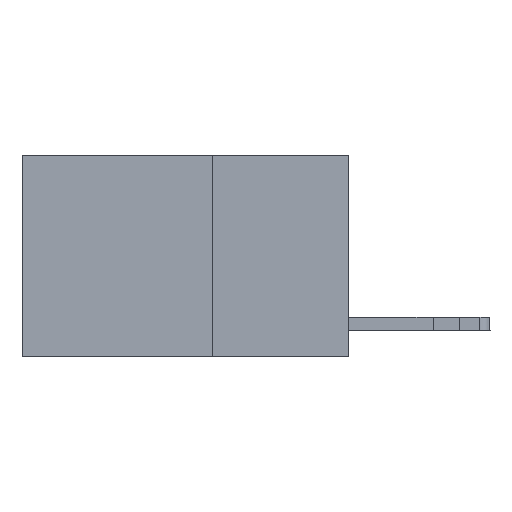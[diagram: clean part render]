
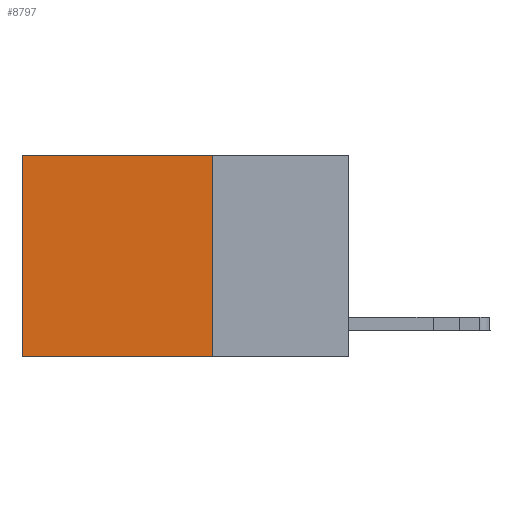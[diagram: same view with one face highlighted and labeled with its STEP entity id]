
A CAD part, left-side view. The second image highlights one B-rep face of the part: STEP entity #8797.
In plain terms, the highlighted planar face has unit normal (-1, 0, 0).
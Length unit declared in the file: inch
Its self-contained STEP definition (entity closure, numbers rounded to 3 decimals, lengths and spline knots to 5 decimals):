
#98 = EDGE_CURVE ( 'NONE', #6494, #3864, #12734, .T. ) ;
#164 = CARTESIAN_POINT ( 'NONE',  ( 0.2625, 0.25, 0. ) ) ;
#440 = DIRECTION ( 'NONE',  ( 0., 0., -1. ) ) ;
#490 = EDGE_CURVE ( 'NONE', #1724, #9659, #8825, .T. ) ;
#713 = DIRECTION ( 'NONE',  ( 0., 1., 0. ) ) ;
#1035 = FACE_OUTER_BOUND ( 'NONE', #4036, .T. ) ;
#1248 = CARTESIAN_POINT ( 'NONE',  ( 0.2625, 0.25, -0.37 ) ) ;
#1346 = CARTESIAN_POINT ( 'NONE',  ( 0.2625, 0.6, 0. ) ) ;
#1724 = VERTEX_POINT ( 'NONE', #13591 ) ;
#2161 = DIRECTION ( 'NONE',  ( 0., 0., -1. ) ) ;
#3864 = VERTEX_POINT ( 'NONE', #1248 ) ;
#4036 = EDGE_LOOP ( 'NONE', ( #8501, #10737, #10221, #10270 ) ) ;
#4062 = VECTOR ( 'NONE', #713, 39.37008 ) ;
#4431 = LINE ( 'NONE', #5503, #10127 ) ;
#4881 = CARTESIAN_POINT ( 'NONE',  ( 0.2625, 0.25, 0. ) ) ;
#5503 = CARTESIAN_POINT ( 'NONE',  ( 0.2625, 0.25, 0. ) ) ;
#6494 = VERTEX_POINT ( 'NONE', #4881 ) ;
#6501 = CARTESIAN_POINT ( 'NONE',  ( 0.2625, 0.6, -0.37 ) ) ;
#6627 = DIRECTION ( 'NONE',  ( 0., 1., 0. ) ) ;
#6655 = VECTOR ( 'NONE', #440, 39.37008 ) ;
#7074 = DIRECTION ( 'NONE',  ( 0., 0., -1. ) ) ;
#8473 = VECTOR ( 'NONE', #2161, 39.37008 ) ;
#8501 = ORIENTED_EDGE ( 'NONE', *, *, #490, .T. ) ;
#8797 = ADVANCED_FACE ( 'NONE', ( #1035 ), #11621, .F. ) ;
#8825 = LINE ( 'NONE', #1346, #8473 ) ;
#9659 = VERTEX_POINT ( 'NONE', #6501 ) ;
#10127 = VECTOR ( 'NONE', #6627, 39.37008 ) ;
#10221 = ORIENTED_EDGE ( 'NONE', *, *, #98, .F. ) ;
#10270 = ORIENTED_EDGE ( 'NONE', *, *, #12315, .T. ) ;
#10737 = ORIENTED_EDGE ( 'NONE', *, *, #12321, .F. ) ;
#11200 = LINE ( 'NONE', #12322, #4062 ) ;
#11621 = PLANE ( 'NONE',  #13851 ) ;
#12315 = EDGE_CURVE ( 'NONE', #6494, #1724, #4431, .T. ) ;
#12321 = EDGE_CURVE ( 'NONE', #3864, #9659, #11200, .T. ) ;
#12322 = CARTESIAN_POINT ( 'NONE',  ( 0.2625, 0.25, -0.37 ) ) ;
#12734 = LINE ( 'NONE', #164, #6655 ) ;
#12768 = CARTESIAN_POINT ( 'NONE',  ( 0.2625, 0.25, 0. ) ) ;
#13591 = CARTESIAN_POINT ( 'NONE',  ( 0.2625, 0.6, 0. ) ) ;
#13851 = AXIS2_PLACEMENT_3D ( 'NONE', #12768, #13918, #7074 ) ;
#13918 = DIRECTION ( 'NONE',  ( 1., 0., 0. ) ) ;
